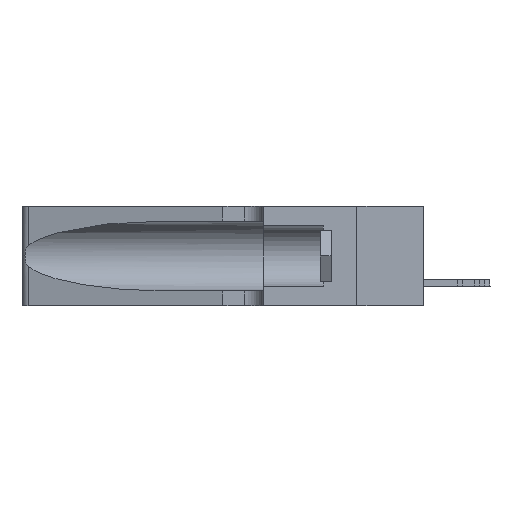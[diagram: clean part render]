
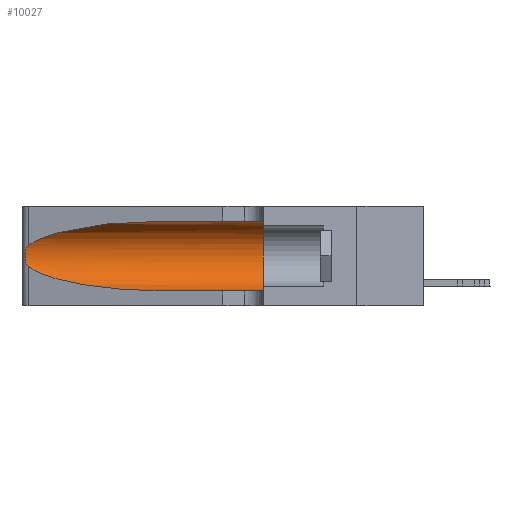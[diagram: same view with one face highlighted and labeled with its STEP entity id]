
A CAD part, left-side view. The second image highlights one B-rep face of the part: STEP entity #10027.
In plain terms, the highlighted cylindrical face has radius 3.308 mm (diameter 6.617 mm), a partial arc.
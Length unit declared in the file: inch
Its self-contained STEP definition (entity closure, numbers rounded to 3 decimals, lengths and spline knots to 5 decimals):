
#153 = CARTESIAN_POINT ( 'NONE',  ( 0.2373, 1.15595, 0.08982 ) ) ;
#378 = ORIENTED_EDGE ( 'NONE', *, *, #21911, .F. ) ;
#472 = LINE ( 'NONE', #4053, #32346 ) ;
#1924 = VERTEX_POINT ( 'NONE', #14117 ) ;
#2349 = EDGE_LOOP ( 'NONE', ( #19825, #41813, #23541, #4778, #13580, #378 ) ) ;
#2536 = EDGE_CURVE ( 'NONE', #39127, #1924, #3781, .T. ) ;
#3091 = CARTESIAN_POINT ( 'NONE',  ( 0.25487, 1.22718, 0.14631 ) ) ;
#3583 = CARTESIAN_POINT ( 'NONE',  ( 0.18966, 0.96281, 0.05475 ) ) ;
#3781 = CIRCLE ( 'NONE', #19580, 0.13025 ) ;
#4007 = VERTEX_POINT ( 'NONE', #41762 ) ;
#4053 = CARTESIAN_POINT ( 'NONE',  ( 0.1305, 1.61858, 0.31525 ) ) ;
#4620 = CARTESIAN_POINT ( 'NONE',  ( 0.26018, 1.23835, 0.19895 ) ) ;
#4778 = ORIENTED_EDGE ( 'NONE', *, *, #6255, .T. ) ;
#5259 = VERTEX_POINT ( 'NONE', #3091 ) ;
#6065 = CARTESIAN_POINT ( 'NONE',  ( 0.1305, 0.72297, 0.31525 ) ) ;
#6255 = EDGE_CURVE ( 'NONE', #12007, #1924, #35307, .T. ) ;
#6755 = CARTESIAN_POINT ( 'NONE',  ( 0.25487, 1.22718, 0.14631 ) ) ;
#7637 =( BOUNDED_CURVE ( )  B_SPLINE_CURVE ( 3, ( #6755, #153, #3583, #29121 ),
 .UNSPECIFIED., .F., .F. ) 
 B_SPLINE_CURVE_WITH_KNOTS ( ( 4, 4 ),
 ( 3.44316, 4.71239 ),
 .UNSPECIFIED. ) 
 CURVE ( )  GEOMETRIC_REPRESENTATION_ITEM ( )  RATIONAL_B_SPLINE_CURVE ( ( 1., 0.87, 0.87, 1. ) ) 
 REPRESENTATION_ITEM ( '' )  );
#7906 = CARTESIAN_POINT ( 'NONE',  ( 0.26075, 1.23896, 0.19203 ) ) ;
#8121 = CARTESIAN_POINT ( 'NONE',  ( 0.1305, 1.61858, 0.185 ) ) ;
#8222 = CARTESIAN_POINT ( 'NONE',  ( 0.25789, 1.23486, 0.15765 ) ) ;
#8223 =( BOUNDED_CURVE ( )  B_SPLINE_CURVE ( 3, ( #6065, #26081, #16306, #12917 ),
 .UNSPECIFIED., .F., .T. ) 
 B_SPLINE_CURVE_WITH_KNOTS ( ( 4, 4 ),
 ( 1.5708, 2.84003 ),
 .UNSPECIFIED. ) 
 CURVE ( )  GEOMETRIC_REPRESENTATION_ITEM ( )  RATIONAL_B_SPLINE_CURVE ( ( 1., 0.87, 0.87, 1. ) ) 
 REPRESENTATION_ITEM ( '' )  );
#8368 = CARTESIAN_POINT ( 'NONE',  ( 0.25487, 1.22718, 0.14631 ) ) ;
#8799 = CARTESIAN_POINT ( 'NONE',  ( 0.25555, 1.22993, 0.14849 ) ) ;
#8899 = EDGE_CURVE ( 'NONE', #18337, #5259, #38093, .T. ) ;
#10027 = ADVANCED_FACE ( 'NONE', ( #27219 ), #14934, .F. ) ;
#11419 = CARTESIAN_POINT ( 'NONE',  ( 0.1305, 0.72297, 0.05475 ) ) ;
#11992 = DIRECTION ( 'NONE',  ( 0., -1., 0. ) ) ;
#12007 = VERTEX_POINT ( 'NONE', #11419 ) ;
#12917 = CARTESIAN_POINT ( 'NONE',  ( 0.25487, 1.22718, 0.22369 ) ) ;
#13159 = AXIS2_PLACEMENT_3D ( 'NONE', #8121, #37581, #28764 ) ;
#13580 = ORIENTED_EDGE ( 'NONE', *, *, #2536, .F. ) ;
#14117 = CARTESIAN_POINT ( 'NONE',  ( 0.1305, 0.35, 0.05475 ) ) ;
#14934 = CYLINDRICAL_SURFACE ( 'NONE', #13159, 0.13025 ) ;
#16306 = CARTESIAN_POINT ( 'NONE',  ( 0.2373, 1.15595, 0.28018 ) ) ;
#17497 = CARTESIAN_POINT ( 'NONE',  ( 0.25639, 1.23184, 0.21858 ) ) ;
#17938 = CARTESIAN_POINT ( 'NONE',  ( 0.26017, 1.23833, 0.17102 ) ) ;
#18079 = CARTESIAN_POINT ( 'NONE',  ( 0.25854, 1.2359, 0.20912 ) ) ;
#18337 = VERTEX_POINT ( 'NONE', #30237 ) ;
#18929 = VECTOR ( 'NONE', #11992, 39.37008 ) ;
#19580 = AXIS2_PLACEMENT_3D ( 'NONE', #34272, #20799, #40696 ) ;
#19825 = ORIENTED_EDGE ( 'NONE', *, *, #30360, .T. ) ;
#20799 = DIRECTION ( 'NONE',  ( 0., 1., 0. ) ) ;
#21789 = CARTESIAN_POINT ( 'NONE',  ( 0.25639, 1.23186, 0.15144 ) ) ;
#21911 = EDGE_CURVE ( 'NONE', #4007, #39127, #472, .T. ) ;
#23541 = ORIENTED_EDGE ( 'NONE', *, *, #39951, .T. ) ;
#24225 = CARTESIAN_POINT ( 'NONE',  ( 0.25787, 1.23484, 0.2124 ) ) ;
#24520 = CARTESIAN_POINT ( 'NONE',  ( 0.25856, 1.23593, 0.16098 ) ) ;
#26081 = CARTESIAN_POINT ( 'NONE',  ( 0.18966, 0.96281, 0.31525 ) ) ;
#27219 = FACE_OUTER_BOUND ( 'NONE', #2349, .T. ) ;
#27249 = CARTESIAN_POINT ( 'NONE',  ( 0.25487, 1.22718, 0.22369 ) ) ;
#28764 = DIRECTION ( 'NONE',  ( 0., 0., -1. ) ) ;
#29121 = CARTESIAN_POINT ( 'NONE',  ( 0.1305, 0.72297, 0.05475 ) ) ;
#30237 = CARTESIAN_POINT ( 'NONE',  ( 0.25487, 1.22718, 0.22369 ) ) ;
#30360 = EDGE_CURVE ( 'NONE', #4007, #18337, #8223, .T. ) ;
#30519 = CARTESIAN_POINT ( 'NONE',  ( 0.25555, 1.22994, 0.2215 ) ) ;
#30962 = CARTESIAN_POINT ( 'NONE',  ( 0.26075, 1.23896, 0.178 ) ) ;
#32346 = VECTOR ( 'NONE', #36945, 39.37008 ) ;
#34272 = CARTESIAN_POINT ( 'NONE',  ( 0.1305, 0.35, 0.185 ) ) ;
#34893 = CARTESIAN_POINT ( 'NONE',  ( 0.1305, 1.61858, 0.05475 ) ) ;
#35307 = LINE ( 'NONE', #34893, #18929 ) ;
#36945 = DIRECTION ( 'NONE',  ( 0., -1., 0. ) ) ;
#37581 = DIRECTION ( 'NONE',  ( 0., -1., 0. ) ) ;
#38093 = B_SPLINE_CURVE_WITH_KNOTS ( 'NONE', 3,
 ( #27249, #30519, #17497, #24225, #18079, #4620, #7906, #30962, #17938, #24520, #8222, #21789, #8799, #8368 ),
 .UNSPECIFIED., .F., .F.,
 ( 4, 2, 2, 2, 2, 2, 4 ),
 ( 0., 0.00027, 0.00053, 0.00107, 0.0016, 0.00187, 0.00214 ),
 .UNSPECIFIED. ) ;
#39127 = VERTEX_POINT ( 'NONE', #40558 ) ;
#39951 = EDGE_CURVE ( 'NONE', #5259, #12007, #7637, .T. ) ;
#40558 = CARTESIAN_POINT ( 'NONE',  ( 0.1305, 0.35, 0.31525 ) ) ;
#40696 = DIRECTION ( 'NONE',  ( 0., 0., 1. ) ) ;
#41762 = CARTESIAN_POINT ( 'NONE',  ( 0.1305, 0.72297, 0.31525 ) ) ;
#41813 = ORIENTED_EDGE ( 'NONE', *, *, #8899, .T. ) ;
